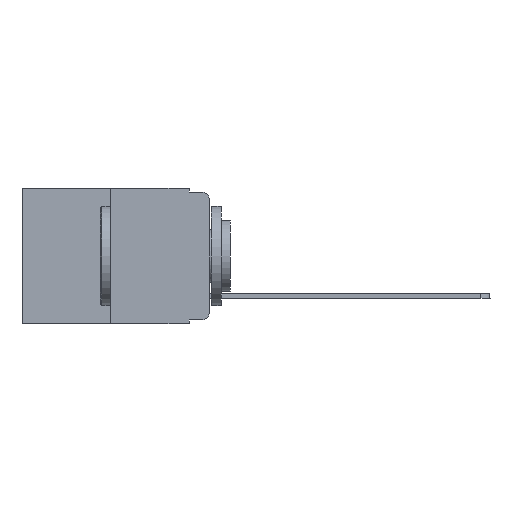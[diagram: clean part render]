
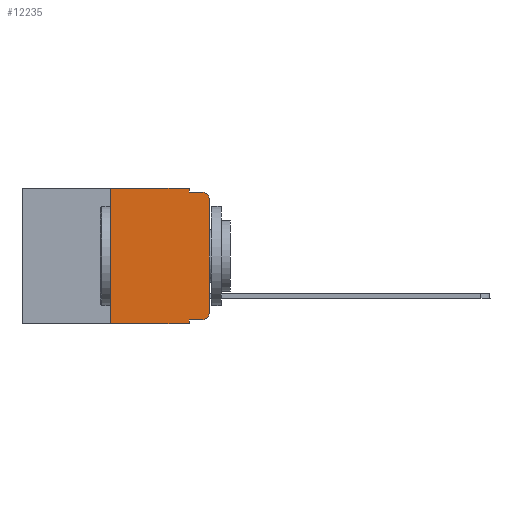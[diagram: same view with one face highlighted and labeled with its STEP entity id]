
A CAD part, left-side view. The second image highlights one B-rep face of the part: STEP entity #12235.
In plain terms, the highlighted planar face has unit normal (-1, 0, 0).
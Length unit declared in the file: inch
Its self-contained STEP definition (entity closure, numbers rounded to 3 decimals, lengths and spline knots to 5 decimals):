
#15 = ORIENTED_EDGE ( 'NONE', *, *, #2109, .F. ) ;
#27 = LINE ( 'NONE', #3562, #19594 ) ;
#64 = CARTESIAN_POINT ( 'NONE',  ( 0., 0.473, -0.343 ) ) ;
#116 = VECTOR ( 'NONE', #11952, 39.37008 ) ;
#426 = EDGE_CURVE ( 'NONE', #4222, #17807, #20423, .T. ) ;
#603 = CARTESIAN_POINT ( 'NONE',  ( 0., 0., -0.03 ) ) ;
#1094 = LINE ( 'NONE', #22418, #12040 ) ;
#1800 = DIRECTION ( 'NONE',  ( 0., 0., -1. ) ) ;
#1876 = AXIS2_PLACEMENT_3D ( 'NONE', #13414, #2111, #4241 ) ;
#1930 = CARTESIAN_POINT ( 'NONE',  ( 0., 0.25, -0.343 ) ) ;
#2109 = EDGE_CURVE ( 'NONE', #10308, #12076, #1094, .T. ) ;
#2111 = DIRECTION ( 'NONE',  ( -1., 0., 0. ) ) ;
#2822 = PLANE ( 'NONE',  #15906 ) ;
#3562 = CARTESIAN_POINT ( 'NONE',  ( 0., 0.051, -0.333 ) ) ;
#3641 = DIRECTION ( 'NONE',  ( 0., -1., 0. ) ) ;
#3772 = DIRECTION ( 'NONE',  ( -1., 0., 0. ) ) ;
#4176 = LINE ( 'NONE', #64, #15975 ) ;
#4222 = VERTEX_POINT ( 'NONE', #6839 ) ;
#4241 = DIRECTION ( 'NONE',  ( 0., 0., -1. ) ) ;
#5181 = LINE ( 'NONE', #21253, #116 ) ;
#5252 = EDGE_CURVE ( 'NONE', #15907, #12830, #27, .T. ) ;
#5369 = EDGE_CURVE ( 'NONE', #10308, #15833, #4176, .T. ) ;
#5677 = CARTESIAN_POINT ( 'NONE',  ( 0., 0.473, 0. ) ) ;
#5966 = ORIENTED_EDGE ( 'NONE', *, *, #12663, .F. ) ;
#6746 = CARTESIAN_POINT ( 'NONE',  ( 0., 0.051, 0. ) ) ;
#6776 = CARTESIAN_POINT ( 'NONE',  ( 0., 0.051, 0. ) ) ;
#6839 = CARTESIAN_POINT ( 'NONE',  ( 0., 0.051, -0.01 ) ) ;
#7850 = ORIENTED_EDGE ( 'NONE', *, *, #11269, .T. ) ;
#9032 = VERTEX_POINT ( 'NONE', #6746 ) ;
#9401 = CIRCLE ( 'NONE', #1876, 0.02 ) ;
#9590 = CARTESIAN_POINT ( 'NONE',  ( 0., 0.02, -0.01 ) ) ;
#9648 = EDGE_CURVE ( 'NONE', #11336, #11630, #5181, .T. ) ;
#10205 = VECTOR ( 'NONE', #22591, 39.37008 ) ;
#10286 = VECTOR ( 'NONE', #22144, 39.37008 ) ;
#10308 = VERTEX_POINT ( 'NONE', #1930 ) ;
#10755 = CARTESIAN_POINT ( 'NONE',  ( 0., 0.02, -0.333 ) ) ;
#10959 = DIRECTION ( 'NONE',  ( 0., 0., 1. ) ) ;
#10961 = CARTESIAN_POINT ( 'NONE',  ( 0., 0.02, -0.313 ) ) ;
#11269 = EDGE_CURVE ( 'NONE', #12830, #11336, #16571, .T. ) ;
#11336 = VERTEX_POINT ( 'NONE', #22338 ) ;
#11630 = VERTEX_POINT ( 'NONE', #603 ) ;
#11928 = CARTESIAN_POINT ( 'NONE',  ( 0., 0.25, 0. ) ) ;
#11952 = DIRECTION ( 'NONE',  ( 0., 0., 1. ) ) ;
#12002 = ORIENTED_EDGE ( 'NONE', *, *, #5252, .T. ) ;
#12040 = VECTOR ( 'NONE', #10959, 39.37008 ) ;
#12076 = VERTEX_POINT ( 'NONE', #11928 ) ;
#12235 = ADVANCED_FACE ( 'NONE', ( #16516 ), #2822, .F. ) ;
#12292 = AXIS2_PLACEMENT_3D ( 'NONE', #10961, #3772, #1800 ) ;
#12663 = EDGE_CURVE ( 'NONE', #9032, #4222, #20678, .T. ) ;
#12830 = VERTEX_POINT ( 'NONE', #10755 ) ;
#12867 = ORIENTED_EDGE ( 'NONE', *, *, #16518, .F. ) ;
#12886 = EDGE_CURVE ( 'NONE', #11630, #17807, #9401, .T. ) ;
#13414 = CARTESIAN_POINT ( 'NONE',  ( 0., 0.02, -0.03 ) ) ;
#14305 = ORIENTED_EDGE ( 'NONE', *, *, #426, .F. ) ;
#14321 = VECTOR ( 'NONE', #19581, 39.37008 ) ;
#14923 = ORIENTED_EDGE ( 'NONE', *, *, #9648, .T. ) ;
#15153 = ORIENTED_EDGE ( 'NONE', *, *, #5369, .T. ) ;
#15793 = LINE ( 'NONE', #5677, #10205 ) ;
#15833 = VERTEX_POINT ( 'NONE', #20472 ) ;
#15906 = AXIS2_PLACEMENT_3D ( 'NONE', #21804, #23527, #21724 ) ;
#15907 = VERTEX_POINT ( 'NONE', #20219 ) ;
#15975 = VECTOR ( 'NONE', #18715, 39.37008 ) ;
#16490 = EDGE_CURVE ( 'NONE', #12076, #9032, #15793, .T. ) ;
#16516 = FACE_OUTER_BOUND ( 'NONE', #20634, .T. ) ;
#16518 = EDGE_CURVE ( 'NONE', #15907, #15833, #23836, .T. ) ;
#16571 = CIRCLE ( 'NONE', #12292, 0.02 ) ;
#16935 = DIRECTION ( 'NONE',  ( 0., -1., 0. ) ) ;
#17807 = VERTEX_POINT ( 'NONE', #9590 ) ;
#18505 = ORIENTED_EDGE ( 'NONE', *, *, #16490, .F. ) ;
#18625 = VECTOR ( 'NONE', #16935, 39.37008 ) ;
#18715 = DIRECTION ( 'NONE',  ( 0., -1., 0. ) ) ;
#19581 = DIRECTION ( 'NONE',  ( 0., 0., -1. ) ) ;
#19594 = VECTOR ( 'NONE', #3641, 39.37008 ) ;
#20143 = ORIENTED_EDGE ( 'NONE', *, *, #12886, .T. ) ;
#20219 = CARTESIAN_POINT ( 'NONE',  ( 0., 0.051, -0.333 ) ) ;
#20423 = LINE ( 'NONE', #20785, #18625 ) ;
#20472 = CARTESIAN_POINT ( 'NONE',  ( 0., 0.051, -0.343 ) ) ;
#20634 = EDGE_LOOP ( 'NONE', ( #14923, #20143, #14305, #5966, #18505, #15, #15153, #12867, #12002, #7850 ) ) ;
#20678 = LINE ( 'NONE', #6776, #10286 ) ;
#20785 = CARTESIAN_POINT ( 'NONE',  ( 0., 0.051, -0.01 ) ) ;
#21253 = CARTESIAN_POINT ( 'NONE',  ( 0., 0., 0. ) ) ;
#21327 = CARTESIAN_POINT ( 'NONE',  ( 0., 0.051, 0. ) ) ;
#21724 = DIRECTION ( 'NONE',  ( 0., 0., -1. ) ) ;
#21804 = CARTESIAN_POINT ( 'NONE',  ( 0., 0.473, 0. ) ) ;
#22144 = DIRECTION ( 'NONE',  ( 0., 0., -1. ) ) ;
#22338 = CARTESIAN_POINT ( 'NONE',  ( 0., 0., -0.313 ) ) ;
#22418 = CARTESIAN_POINT ( 'NONE',  ( 0., 0.25, 0. ) ) ;
#22591 = DIRECTION ( 'NONE',  ( 0., -1., 0. ) ) ;
#23527 = DIRECTION ( 'NONE',  ( 1., 0., 0. ) ) ;
#23836 = LINE ( 'NONE', #21327, #14321 ) ;
